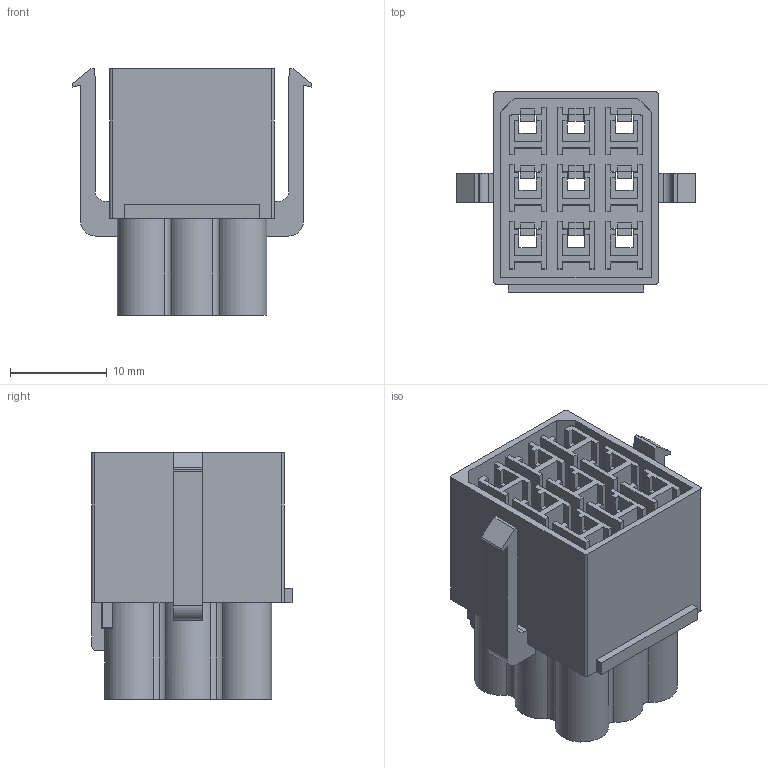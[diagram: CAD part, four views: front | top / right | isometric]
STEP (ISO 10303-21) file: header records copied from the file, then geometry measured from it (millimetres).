
FILE_DESCRIPTION (( 'STEP AP214' ), '1' );
FILE_NAME ('567-009-000-410.STEP', '2020-07-27T20:22:10', ( '' ), ( '' ), 'SwSTEP 2.0', 'SolidWorks 2020', '' );
FILE_SCHEMA (( 'AUTOMOTIVE_DESIGN' ));
Length unit declared in the file: millimetre
Products named in the file (1): 567-009-000-410
Bounding box: 24.8 x 20.7 x 25.5 mm (x, y, z)
Volume: 3053.5 mm3; surface area: 9148 mm2
Topology: 1 solids, 1 shells, 669 faces, 1913 edges, 1266 vertices
Faces by surface type: plane 545, cylinder 101, bspline 21, sphere 2
Entity records: 22675 total; most frequent: CARTESIAN_POINT 5226, ORIENTED_EDGE 3822, DIRECTION 3337, EDGE_CURVE 1911, LINE 1587, VECTOR 1587, VERTEX_POINT 1266, AXIS2_PLACEMENT_3D 875
